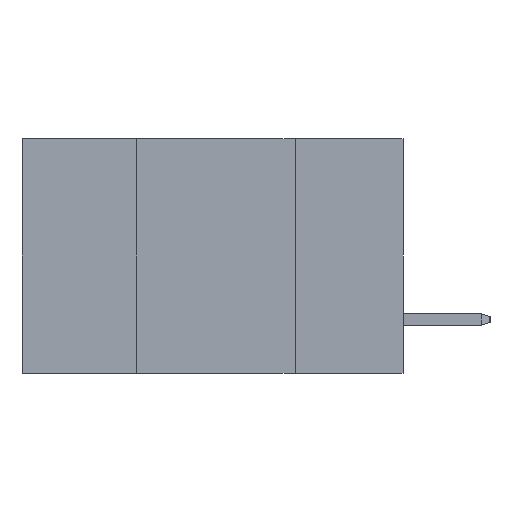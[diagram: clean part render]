
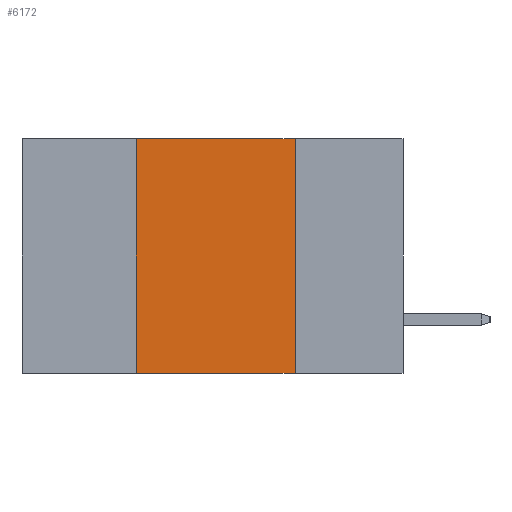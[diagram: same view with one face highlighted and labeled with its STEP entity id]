
A CAD part, left-side view. The second image highlights one B-rep face of the part: STEP entity #6172.
In plain terms, the highlighted planar face has unit normal (-1, 0, 0).
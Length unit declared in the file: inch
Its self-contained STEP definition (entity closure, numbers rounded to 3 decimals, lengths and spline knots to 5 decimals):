
#251 = DIRECTION ( 'NONE',  ( 0., -1., 0. ) ) ;
#373 = CARTESIAN_POINT ( 'NONE',  ( 0., 0.42, 0. ) ) ;
#686 = VECTOR ( 'NONE', #3384, 39.37008 ) ;
#811 = VECTOR ( 'NONE', #9638, 39.37008 ) ;
#1108 = CARTESIAN_POINT ( 'NONE',  ( 0., 0.42, 0. ) ) ;
#1166 = EDGE_LOOP ( 'NONE', ( #11164, #2323, #3645, #2958 ) ) ;
#1217 = VERTEX_POINT ( 'NONE', #6653 ) ;
#1581 = EDGE_CURVE ( 'NONE', #12760, #1217, #9370, .T. ) ;
#2323 = ORIENTED_EDGE ( 'NONE', *, *, #9674, .F. ) ;
#2775 = DIRECTION ( 'NONE',  ( 0., 0., -1. ) ) ;
#2958 = ORIENTED_EDGE ( 'NONE', *, *, #4952, .T. ) ;
#3133 = CARTESIAN_POINT ( 'NONE',  ( 0., 0.17, 0. ) ) ;
#3384 = DIRECTION ( 'NONE',  ( 0., 0., 1. ) ) ;
#3645 = ORIENTED_EDGE ( 'NONE', *, *, #8364, .F. ) ;
#4592 = AXIS2_PLACEMENT_3D ( 'NONE', #6153, #11838, #2775 ) ;
#4952 = EDGE_CURVE ( 'NONE', #7246, #1217, #4958, .T. ) ;
#4958 = LINE ( 'NONE', #14135, #811 ) ;
#5068 = FACE_OUTER_BOUND ( 'NONE', #1166, .T. ) ;
#6153 = CARTESIAN_POINT ( 'NONE',  ( 0., 0.6, 0. ) ) ;
#6172 = ADVANCED_FACE ( 'NONE', ( #5068 ), #12137, .F. ) ;
#6333 = CARTESIAN_POINT ( 'NONE',  ( 0., 0.6, 0. ) ) ;
#6653 = CARTESIAN_POINT ( 'NONE',  ( 0., 0.17, -0.37 ) ) ;
#7246 = VERTEX_POINT ( 'NONE', #11829 ) ;
#7577 = VERTEX_POINT ( 'NONE', #1108 ) ;
#8364 = EDGE_CURVE ( 'NONE', #7246, #7577, #12743, .T. ) ;
#9370 = LINE ( 'NONE', #14091, #12052 ) ;
#9638 = DIRECTION ( 'NONE',  ( 0., -1., 0. ) ) ;
#9674 = EDGE_CURVE ( 'NONE', #7577, #12760, #10726, .T. ) ;
#10726 = LINE ( 'NONE', #6333, #12745 ) ;
#11164 = ORIENTED_EDGE ( 'NONE', *, *, #1581, .F. ) ;
#11829 = CARTESIAN_POINT ( 'NONE',  ( 0., 0.42, -0.37 ) ) ;
#11838 = DIRECTION ( 'NONE',  ( 1., 0., 0. ) ) ;
#12052 = VECTOR ( 'NONE', #13783, 39.37008 ) ;
#12137 = PLANE ( 'NONE',  #4592 ) ;
#12743 = LINE ( 'NONE', #373, #686 ) ;
#12745 = VECTOR ( 'NONE', #251, 39.37008 ) ;
#12760 = VERTEX_POINT ( 'NONE', #3133 ) ;
#13783 = DIRECTION ( 'NONE',  ( 0., 0., -1. ) ) ;
#14091 = CARTESIAN_POINT ( 'NONE',  ( 0., 0.17, 0. ) ) ;
#14135 = CARTESIAN_POINT ( 'NONE',  ( 0., 0.6, -0.37 ) ) ;
